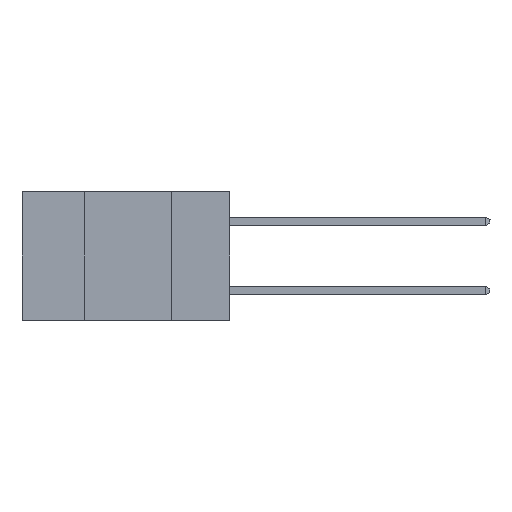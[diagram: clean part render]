
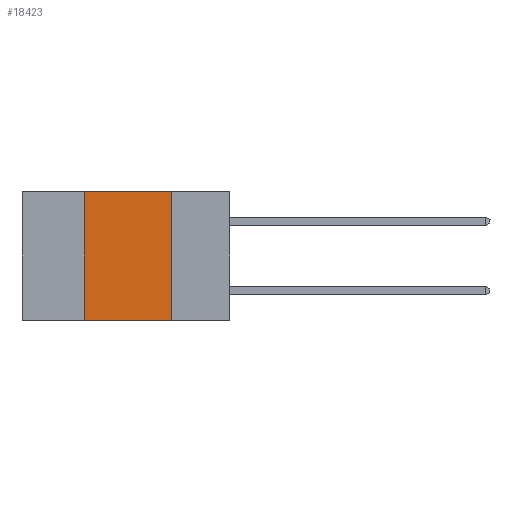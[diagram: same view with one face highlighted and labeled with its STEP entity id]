
A CAD part, left-side view. The second image highlights one B-rep face of the part: STEP entity #18423.
In plain terms, the highlighted planar face has unit normal (-1, 0, 0).
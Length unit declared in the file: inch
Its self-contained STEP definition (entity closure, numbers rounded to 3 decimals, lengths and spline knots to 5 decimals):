
#137 = ORIENTED_EDGE ( 'NONE', *, *, #4496, .F. ) ;
#467 = EDGE_CURVE ( 'NONE', #10195, #3372, #1640, .T. ) ;
#954 = LINE ( 'NONE', #4909, #12366 ) ;
#1640 = LINE ( 'NONE', #11468, #15966 ) ;
#2792 = ORIENTED_EDGE ( 'NONE', *, *, #13794, .T. ) ;
#3263 = DIRECTION ( 'NONE',  ( 0., -1., 0. ) ) ;
#3372 = VERTEX_POINT ( 'NONE', #8855 ) ;
#3484 = DIRECTION ( 'NONE',  ( 1., 0., 0. ) ) ;
#3502 = CARTESIAN_POINT ( 'NONE',  ( 0., 0.17, 0. ) ) ;
#4301 = CARTESIAN_POINT ( 'NONE',  ( 0., 0.6, -0.37 ) ) ;
#4496 = EDGE_CURVE ( 'NONE', #15943, #17371, #17521, .T. ) ;
#4617 = CARTESIAN_POINT ( 'NONE',  ( 0., 0.42, -0.37 ) ) ;
#4632 = ORIENTED_EDGE ( 'NONE', *, *, #11622, .F. ) ;
#4909 = CARTESIAN_POINT ( 'NONE',  ( 0., 0.6, 0. ) ) ;
#7816 = DIRECTION ( 'NONE',  ( 0., 0., -1. ) ) ;
#8855 = CARTESIAN_POINT ( 'NONE',  ( 0., 0.17, -0.37 ) ) ;
#9759 = CARTESIAN_POINT ( 'NONE',  ( 0., 0.42, -0.37 ) ) ;
#10195 = VERTEX_POINT ( 'NONE', #3502 ) ;
#10361 = DIRECTION ( 'NONE',  ( 0., 0., 1. ) ) ;
#10540 = EDGE_LOOP ( 'NONE', ( #13801, #4632, #137, #2792 ) ) ;
#11093 = AXIS2_PLACEMENT_3D ( 'NONE', #12244, #3484, #7816 ) ;
#11468 = CARTESIAN_POINT ( 'NONE',  ( 0., 0.17, -0.37 ) ) ;
#11482 = CARTESIAN_POINT ( 'NONE',  ( 0., 0.42, 0. ) ) ;
#11622 = EDGE_CURVE ( 'NONE', #17371, #10195, #954, .T. ) ;
#12069 = DIRECTION ( 'NONE',  ( 0., -1., 0. ) ) ;
#12244 = CARTESIAN_POINT ( 'NONE',  ( 0., 0.6, 0. ) ) ;
#12366 = VECTOR ( 'NONE', #12069, 39.37008 ) ;
#13794 = EDGE_CURVE ( 'NONE', #15943, #3372, #17213, .T. ) ;
#13801 = ORIENTED_EDGE ( 'NONE', *, *, #467, .F. ) ;
#15544 = VECTOR ( 'NONE', #3263, 39.37008 ) ;
#15943 = VERTEX_POINT ( 'NONE', #9759 ) ;
#15966 = VECTOR ( 'NONE', #17211, 39.37008 ) ;
#16389 = FACE_OUTER_BOUND ( 'NONE', #10540, .T. ) ;
#16593 = PLANE ( 'NONE',  #11093 ) ;
#17211 = DIRECTION ( 'NONE',  ( 0., 0., -1. ) ) ;
#17213 = LINE ( 'NONE', #4301, #15544 ) ;
#17371 = VERTEX_POINT ( 'NONE', #11482 ) ;
#17521 = LINE ( 'NONE', #4617, #18007 ) ;
#18007 = VECTOR ( 'NONE', #10361, 39.37008 ) ;
#18423 = ADVANCED_FACE ( 'NONE', ( #16389 ), #16593, .F. ) ;
